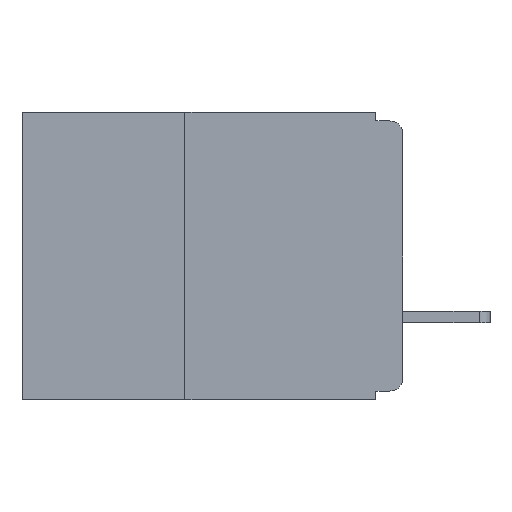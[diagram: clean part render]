
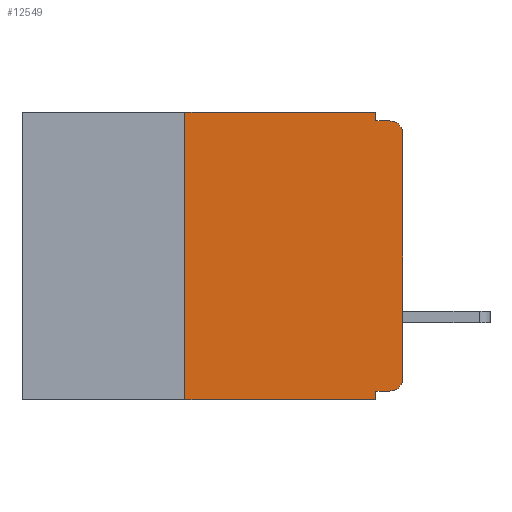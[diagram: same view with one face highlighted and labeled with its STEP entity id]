
A CAD part, left-side view. The second image highlights one B-rep face of the part: STEP entity #12549.
In plain terms, the highlighted planar face has unit normal (-1, 0, 0).
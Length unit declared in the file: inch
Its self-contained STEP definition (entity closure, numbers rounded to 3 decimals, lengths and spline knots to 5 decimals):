
#825 = VERTEX_POINT ( 'NONE', #4056 ) ;
#1318 = CIRCLE ( 'NONE', #17747, 0.015 ) ;
#1523 = VERTEX_POINT ( 'NONE', #14881 ) ;
#1770 = ORIENTED_EDGE ( 'NONE', *, *, #3465, .F. ) ;
#2793 = ORIENTED_EDGE ( 'NONE', *, *, #9984, .F. ) ;
#3465 = EDGE_CURVE ( 'NONE', #11602, #7585, #9655, .T. ) ;
#3593 = LINE ( 'NONE', #5097, #3703 ) ;
#3703 = VECTOR ( 'NONE', #5394, 39.37008 ) ;
#3920 = DIRECTION ( 'NONE',  ( 0., 0., -1. ) ) ;
#3994 = PLANE ( 'NONE',  #15477 ) ;
#4023 = CARTESIAN_POINT ( 'NONE',  ( 0., 0.437, 0. ) ) ;
#4056 = CARTESIAN_POINT ( 'NONE',  ( 0., 0.031, -0.32 ) ) ;
#4205 = DIRECTION ( 'NONE',  ( 1., 0., 0. ) ) ;
#4459 = VECTOR ( 'NONE', #11213, 39.37008 ) ;
#4463 = VECTOR ( 'NONE', #14133, 39.37008 ) ;
#4490 = CARTESIAN_POINT ( 'NONE',  ( 0., 0., -0.025 ) ) ;
#4517 = LINE ( 'NONE', #10755, #4459 ) ;
#5086 = ORIENTED_EDGE ( 'NONE', *, *, #11986, .T. ) ;
#5097 = CARTESIAN_POINT ( 'NONE',  ( 0., 0.25, -0.33 ) ) ;
#5362 = VERTEX_POINT ( 'NONE', #6483 ) ;
#5394 = DIRECTION ( 'NONE',  ( 0., 0., 1. ) ) ;
#5560 = CARTESIAN_POINT ( 'NONE',  ( 0., 0.031, -0.01 ) ) ;
#5902 = VERTEX_POINT ( 'NONE', #4490 ) ;
#6028 = CARTESIAN_POINT ( 'NONE',  ( 0., 0.25, -0.33 ) ) ;
#6074 = CARTESIAN_POINT ( 'NONE',  ( 0., 0.015, -0.01 ) ) ;
#6117 = CARTESIAN_POINT ( 'NONE',  ( 0., 0., -0.305 ) ) ;
#6274 = VERTEX_POINT ( 'NONE', #15373 ) ;
#6483 = CARTESIAN_POINT ( 'NONE',  ( 0., 0.015, -0.32 ) ) ;
#6989 = VECTOR ( 'NONE', #15677, 39.37008 ) ;
#7106 = ORIENTED_EDGE ( 'NONE', *, *, #12393, .F. ) ;
#7532 = VERTEX_POINT ( 'NONE', #6117 ) ;
#7585 = VERTEX_POINT ( 'NONE', #6074 ) ;
#7797 = CARTESIAN_POINT ( 'NONE',  ( 0., 0.437, 0. ) ) ;
#7871 = ORIENTED_EDGE ( 'NONE', *, *, #13857, .F. ) ;
#8020 = LINE ( 'NONE', #7797, #6989 ) ;
#8120 = DIRECTION ( 'NONE',  ( 0., 0., 1. ) ) ;
#8772 = ORIENTED_EDGE ( 'NONE', *, *, #11451, .F. ) ;
#8991 = EDGE_LOOP ( 'NONE', ( #14796, #16709, #1770, #2793, #8772, #14586, #5086, #7106, #7871, #9019 ) ) ;
#9019 = ORIENTED_EDGE ( 'NONE', *, *, #18024, .T. ) ;
#9026 = LINE ( 'NONE', #11243, #15791 ) ;
#9309 = LINE ( 'NONE', #17736, #4463 ) ;
#9420 = CARTESIAN_POINT ( 'NONE',  ( 0., 0., 0. ) ) ;
#9633 = VECTOR ( 'NONE', #12092, 39.37008 ) ;
#9655 = LINE ( 'NONE', #12447, #9633 ) ;
#9984 = EDGE_CURVE ( 'NONE', #15887, #11602, #4517, .T. ) ;
#10157 = VERTEX_POINT ( 'NONE', #6028 ) ;
#10199 = EDGE_CURVE ( 'NONE', #10157, #1523, #3593, .T. ) ;
#10755 = CARTESIAN_POINT ( 'NONE',  ( 0., 0.031, 0. ) ) ;
#11073 = FACE_OUTER_BOUND ( 'NONE', #8991, .T. ) ;
#11213 = DIRECTION ( 'NONE',  ( 0., 0., -1. ) ) ;
#11216 = DIRECTION ( 'NONE',  ( 0., 1., 0. ) ) ;
#11243 = CARTESIAN_POINT ( 'NONE',  ( 0., 0., -0.32 ) ) ;
#11290 = AXIS2_PLACEMENT_3D ( 'NONE', #11927, #12623, #12570 ) ;
#11451 = EDGE_CURVE ( 'NONE', #1523, #15887, #8020, .T. ) ;
#11602 = VERTEX_POINT ( 'NONE', #5560 ) ;
#11927 = CARTESIAN_POINT ( 'NONE',  ( 0., 0.015, -0.025 ) ) ;
#11974 = CARTESIAN_POINT ( 'NONE',  ( 0., 0.031, 0. ) ) ;
#11986 = EDGE_CURVE ( 'NONE', #10157, #6274, #17393, .T. ) ;
#12092 = DIRECTION ( 'NONE',  ( 0., -1., 0. ) ) ;
#12178 = DIRECTION ( 'NONE',  ( -1., 0., 0. ) ) ;
#12198 = DIRECTION ( 'NONE',  ( 0., 0., -1. ) ) ;
#12218 = CARTESIAN_POINT ( 'NONE',  ( 0., 0.015, -0.305 ) ) ;
#12393 = EDGE_CURVE ( 'NONE', #825, #6274, #9309, .T. ) ;
#12447 = CARTESIAN_POINT ( 'NONE',  ( 0., 0., -0.01 ) ) ;
#12549 = ADVANCED_FACE ( 'NONE', ( #11073 ), #3994, .F. ) ;
#12569 = DIRECTION ( 'NONE',  ( 0., -1., 0. ) ) ;
#12570 = DIRECTION ( 'NONE',  ( 0., 0., -1. ) ) ;
#12623 = DIRECTION ( 'NONE',  ( -1., 0., 0. ) ) ;
#12976 = CARTESIAN_POINT ( 'NONE',  ( 0., 0.437, -0.33 ) ) ;
#13516 = EDGE_CURVE ( 'NONE', #5902, #7585, #16056, .T. ) ;
#13857 = EDGE_CURVE ( 'NONE', #5362, #825, #9026, .T. ) ;
#14133 = DIRECTION ( 'NONE',  ( 0., 0., -1. ) ) ;
#14586 = ORIENTED_EDGE ( 'NONE', *, *, #10199, .F. ) ;
#14796 = ORIENTED_EDGE ( 'NONE', *, *, #15898, .T. ) ;
#14845 = VECTOR ( 'NONE', #8120, 39.37008 ) ;
#14881 = CARTESIAN_POINT ( 'NONE',  ( 0., 0.25, 0. ) ) ;
#14921 = LINE ( 'NONE', #9420, #14845 ) ;
#15373 = CARTESIAN_POINT ( 'NONE',  ( 0., 0.031, -0.33 ) ) ;
#15477 = AXIS2_PLACEMENT_3D ( 'NONE', #4023, #4205, #3920 ) ;
#15677 = DIRECTION ( 'NONE',  ( 0., -1., 0. ) ) ;
#15791 = VECTOR ( 'NONE', #11216, 39.37008 ) ;
#15887 = VERTEX_POINT ( 'NONE', #11974 ) ;
#15898 = EDGE_CURVE ( 'NONE', #7532, #5902, #14921, .T. ) ;
#16056 = CIRCLE ( 'NONE', #11290, 0.015 ) ;
#16709 = ORIENTED_EDGE ( 'NONE', *, *, #13516, .T. ) ;
#16997 = VECTOR ( 'NONE', #12569, 39.37008 ) ;
#17393 = LINE ( 'NONE', #12976, #16997 ) ;
#17736 = CARTESIAN_POINT ( 'NONE',  ( 0., 0.031, -0.33 ) ) ;
#17747 = AXIS2_PLACEMENT_3D ( 'NONE', #12218, #12178, #12198 ) ;
#18024 = EDGE_CURVE ( 'NONE', #5362, #7532, #1318, .T. ) ;
